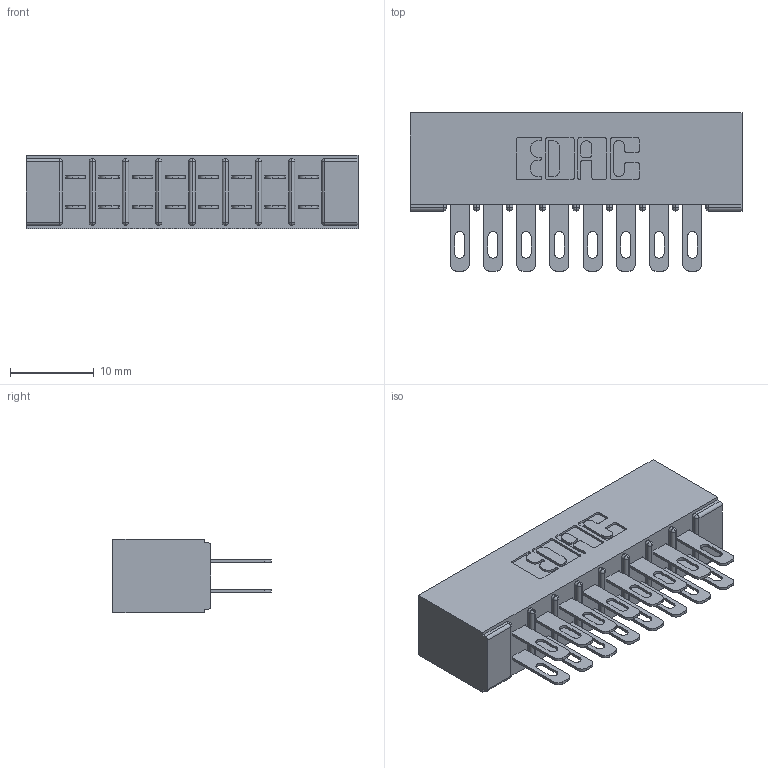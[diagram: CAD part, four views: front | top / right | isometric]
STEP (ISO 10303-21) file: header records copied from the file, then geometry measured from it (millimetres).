
FILE_DESCRIPTION (( 'STEP AP203' ), '1' );
FILE_NAME ('355-016-500-501.STEP', '2019-09-11T01:48:29', ( '' ), ( '' ), 'SwSTEP 2.0', 'SolidWorks 2016', '' );
FILE_SCHEMA (( 'CONFIG_CONTROL_DESIGN' ));
Length unit declared in the file: inch
Products named in the file (3): 305-290-001_500; 355-016-500-501; 305 Part_No Mounting
Assembly tree (17 placements, depth 2):
  355-016-500-501
    305 Part_No Mounting
    305-290-001_500  x16
Bounding box: 39.57 x 18.85 x 8.71 mm (x, y, z)
Volume: 2624.5 mm3; surface area: 5251.4 mm2
Topology: 17 solids, 17 shells, 908 faces, 2588 edges, 1680 vertices
Faces by surface type: plane 512, cylinder 364, sphere 32
Entity records: 12545 total; most frequent: CARTESIAN_POINT 2074, ORIENTED_EDGE 2052, DIRECTION 2034, EDGE_CURVE 1026, VECTOR 794, LINE 794, VERTEX_POINT 660, AXIS2_PLACEMENT_3D 620
